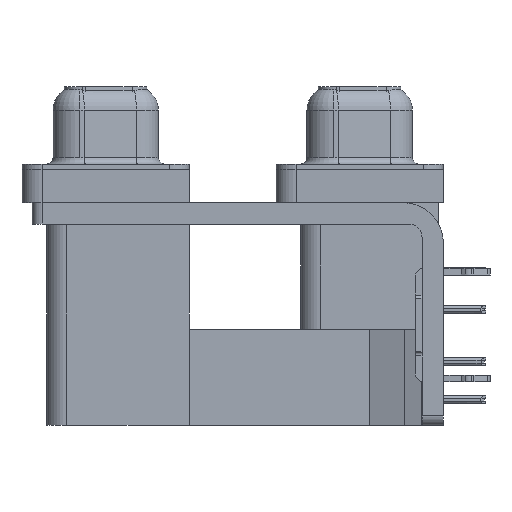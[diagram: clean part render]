
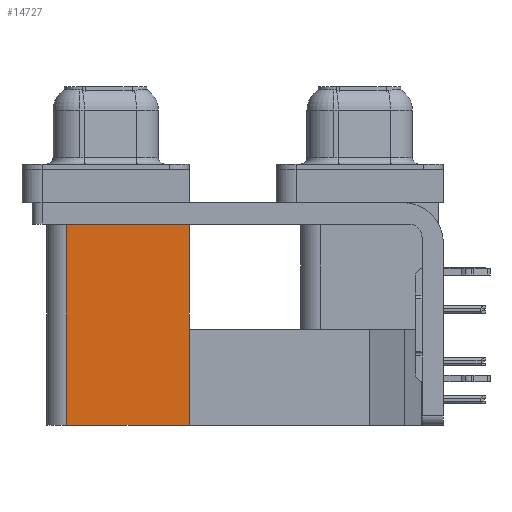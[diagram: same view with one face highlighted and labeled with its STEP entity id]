
A CAD part, left-side view. The second image highlights one B-rep face of the part: STEP entity #14727.
In plain terms, the highlighted planar face has unit normal (-1, 0, 0).
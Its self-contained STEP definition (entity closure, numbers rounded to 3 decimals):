
#495 = LINE ( 'NONE', #10964, #23836 ) ;
#783 = VERTEX_POINT ( 'NONE', #8280 ) ;
#1762 = DIRECTION ( 'NONE',  ( 0., 1., 0. ) ) ;
#2023 = VERTEX_POINT ( 'NONE', #29244 ) ;
#3612 = CARTESIAN_POINT ( 'NONE',  ( 3.79, 12.775, -19.2 ) ) ;
#4559 = AXIS2_PLACEMENT_3D ( 'NONE', #9116, #22148, #1762 ) ;
#5773 = DIRECTION ( 'NONE',  ( 0., 1., 0. ) ) ;
#8280 = CARTESIAN_POINT ( 'NONE',  ( 3.79, 21.975, -2.5 ) ) ;
#8320 = VERTEX_POINT ( 'NONE', #21138 ) ;
#8962 = CARTESIAN_POINT ( 'NONE',  ( 3.79, 12.775, -19.2 ) ) ;
#9116 = CARTESIAN_POINT ( 'NONE',  ( 3.79, 12.775, -19.2 ) ) ;
#10964 = CARTESIAN_POINT ( 'NONE',  ( 3.79, 21.975, -19.2 ) ) ;
#12238 = ORIENTED_EDGE ( 'NONE', *, *, #36610, .T. ) ;
#12247 = ORIENTED_EDGE ( 'NONE', *, *, #21383, .F. ) ;
#13209 = VECTOR ( 'NONE', #22216, 1000. ) ;
#14727 = ADVANCED_FACE ( 'NONE', ( #41578 ), #25357, .F. ) ;
#15403 = LINE ( 'NONE', #25227, #30352 ) ;
#21138 = CARTESIAN_POINT ( 'NONE',  ( 3.79, 21.975, -19.2 ) ) ;
#21383 = EDGE_CURVE ( 'NONE', #21786, #8320, #21788, .T. ) ;
#21786 = VERTEX_POINT ( 'NONE', #39474 ) ;
#21788 = LINE ( 'NONE', #8962, #36282 ) ;
#22148 = DIRECTION ( 'NONE',  ( 1., 0., 0. ) ) ;
#22216 = DIRECTION ( 'NONE',  ( 0., 0., 1. ) ) ;
#23022 = EDGE_LOOP ( 'NONE', ( #35878, #41926, #12247, #12238 ) ) ;
#23836 = VECTOR ( 'NONE', #24007, 1000. ) ;
#24007 = DIRECTION ( 'NONE',  ( 0., 0., 1. ) ) ;
#25227 = CARTESIAN_POINT ( 'NONE',  ( 3.79, 12.775, -2.5 ) ) ;
#25357 = PLANE ( 'NONE',  #4559 ) ;
#27506 = EDGE_CURVE ( 'NONE', #2023, #783, #15403, .T. ) ;
#29244 = CARTESIAN_POINT ( 'NONE',  ( 3.79, 12.775, -2.5 ) ) ;
#30352 = VECTOR ( 'NONE', #5773, 1000. ) ;
#33212 = EDGE_CURVE ( 'NONE', #8320, #783, #495, .T. ) ;
#34390 = DIRECTION ( 'NONE',  ( 0., 1., 0. ) ) ;
#35231 = LINE ( 'NONE', #3612, #13209 ) ;
#35878 = ORIENTED_EDGE ( 'NONE', *, *, #27506, .T. ) ;
#36282 = VECTOR ( 'NONE', #34390, 1000. ) ;
#36610 = EDGE_CURVE ( 'NONE', #21786, #2023, #35231, .T. ) ;
#39474 = CARTESIAN_POINT ( 'NONE',  ( 3.79, 12.775, -19.2 ) ) ;
#41578 = FACE_OUTER_BOUND ( 'NONE', #23022, .T. ) ;
#41926 = ORIENTED_EDGE ( 'NONE', *, *, #33212, .F. ) ;
